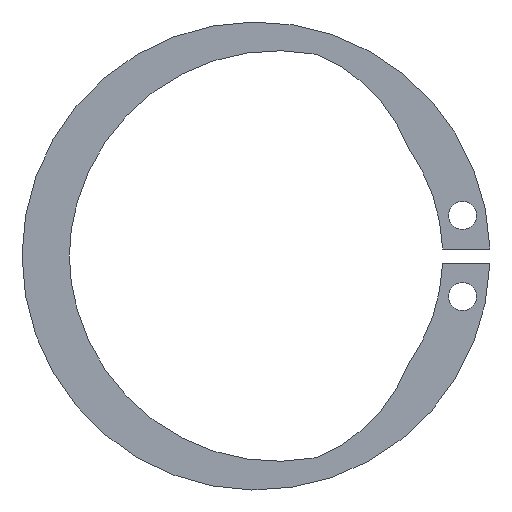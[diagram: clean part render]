
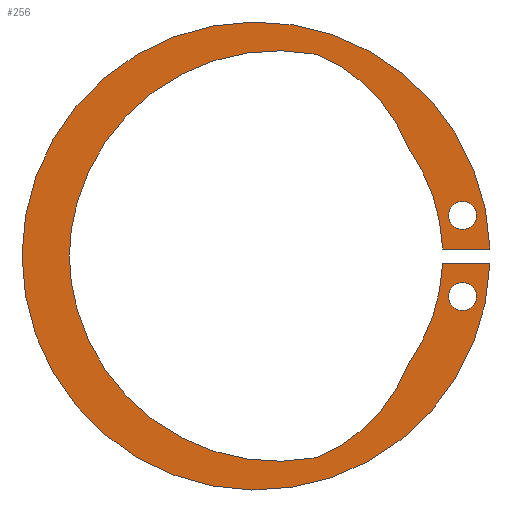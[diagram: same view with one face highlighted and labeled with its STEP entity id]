
A CAD part, front view. The second image highlights one B-rep face of the part: STEP entity #256.
In plain terms, the highlighted planar face has unit normal (0, -1, 0).
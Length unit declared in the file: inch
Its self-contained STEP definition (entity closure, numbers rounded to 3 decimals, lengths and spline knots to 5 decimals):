
#18=PLANE('',#310);
#21=LINE('',#417,#35);
#31=LINE('',#464,#45);
#35=VECTOR('',#335,0.3937);
#45=VECTOR('',#389,0.3937);
#51=FACE_BOUND('',#85,.T.);
#52=FACE_BOUND('',#86,.T.);
#66=FACE_OUTER_BOUND('',#84,.T.);
#84=EDGE_LOOP('',(#221,#222,#223,#224,#225,#226,#227,#228,#229,#230));
#85=EDGE_LOOP('',(#231));
#86=EDGE_LOOP('',(#232));
#88=CIRCLE('',#279,0.05);
#90=CIRCLE('',#282,0.05);
#91=CIRCLE('',#284,0.8355);
#93=CIRCLE('',#288,0.6665);
#95=CIRCLE('',#291,0.57967);
#97=CIRCLE('',#294,0.74404);
#99=CIRCLE('',#297,0.6665);
#101=CIRCLE('',#300,0.74404);
#103=CIRCLE('',#303,0.57967);
#105=CIRCLE('',#306,0.6665);
#108=VERTEX_POINT('',#399);
#110=VERTEX_POINT('',#404);
#111=VERTEX_POINT('',#407);
#112=VERTEX_POINT('',#408);
#115=VERTEX_POINT('',#416);
#117=VERTEX_POINT('',#422);
#119=VERTEX_POINT('',#428);
#121=VERTEX_POINT('',#434);
#123=VERTEX_POINT('',#440);
#125=VERTEX_POINT('',#446);
#127=VERTEX_POINT('',#452);
#129=VERTEX_POINT('',#458);
#132=EDGE_CURVE('',#108,#108,#88,.T.);
#134=EDGE_CURVE('',#110,#110,#90,.T.);
#135=EDGE_CURVE('',#111,#112,#91,.T.);
#139=EDGE_CURVE('',#115,#111,#21,.T.);
#142=EDGE_CURVE('',#117,#115,#93,.T.);
#145=EDGE_CURVE('',#119,#117,#95,.T.);
#148=EDGE_CURVE('',#121,#119,#97,.T.);
#151=EDGE_CURVE('',#123,#121,#99,.T.);
#154=EDGE_CURVE('',#125,#123,#101,.T.);
#157=EDGE_CURVE('',#127,#125,#103,.T.);
#160=EDGE_CURVE('',#129,#127,#105,.T.);
#163=EDGE_CURVE('',#112,#129,#31,.T.);
#221=ORIENTED_EDGE('',*,*,#163,.F.);
#222=ORIENTED_EDGE('',*,*,#135,.F.);
#223=ORIENTED_EDGE('',*,*,#139,.F.);
#224=ORIENTED_EDGE('',*,*,#142,.F.);
#225=ORIENTED_EDGE('',*,*,#145,.F.);
#226=ORIENTED_EDGE('',*,*,#148,.F.);
#227=ORIENTED_EDGE('',*,*,#151,.F.);
#228=ORIENTED_EDGE('',*,*,#154,.F.);
#229=ORIENTED_EDGE('',*,*,#157,.F.);
#230=ORIENTED_EDGE('',*,*,#160,.F.);
#231=ORIENTED_EDGE('',*,*,#132,.T.);
#232=ORIENTED_EDGE('',*,*,#134,.T.);
#256=ADVANCED_FACE('',(#66,#51,#52),#18,.F.);
#279=AXIS2_PLACEMENT_3D('',#400,#317,#318);
#282=AXIS2_PLACEMENT_3D('',#405,#323,#324);
#284=AXIS2_PLACEMENT_3D('',#409,#327,#328);
#288=AXIS2_PLACEMENT_3D('',#423,#340,#341);
#291=AXIS2_PLACEMENT_3D('',#429,#347,#348);
#294=AXIS2_PLACEMENT_3D('',#435,#354,#355);
#297=AXIS2_PLACEMENT_3D('',#441,#361,#362);
#300=AXIS2_PLACEMENT_3D('',#447,#368,#369);
#303=AXIS2_PLACEMENT_3D('',#453,#375,#376);
#306=AXIS2_PLACEMENT_3D('',#459,#382,#383);
#310=AXIS2_PLACEMENT_3D('',#467,#393,#394);
#317=DIRECTION('center_axis',(0.,1.,0.));
#318=DIRECTION('ref_axis',(1.,0.,0.));
#323=DIRECTION('center_axis',(0.,1.,0.));
#324=DIRECTION('ref_axis',(1.,0.,0.));
#327=DIRECTION('center_axis',(0.,1.,0.));
#328=DIRECTION('ref_axis',(0.999,0.,-0.033));
#335=DIRECTION('',(1.,0.,-0.017));
#340=DIRECTION('center_axis',(0.,-1.,0.));
#341=DIRECTION('ref_axis',(-0.999,0.,0.038));
#347=DIRECTION('center_axis',(0.,-1.,0.));
#348=DIRECTION('ref_axis',(-0.935,0.,0.354));
#354=DIRECTION('center_axis',(0.,-1.,0.));
#355=DIRECTION('ref_axis',(-0.184,0.,0.983));
#361=DIRECTION('center_axis',(0.,-1.,0.));
#362=DIRECTION('ref_axis',(0.96,0.,0.279));
#368=DIRECTION('center_axis',(0.,-1.,0.));
#369=DIRECTION('ref_axis',(1.,0.,-0.015));
#375=DIRECTION('center_axis',(0.,-1.,0.));
#376=DIRECTION('ref_axis',(-0.368,0.,-0.93));
#382=DIRECTION('center_axis',(0.,-1.,0.));
#383=DIRECTION('ref_axis',(-0.815,0.,-0.58));
#389=DIRECTION('',(-1.,0.,0.));
#393=DIRECTION('center_axis',(0.,1.,0.));
#394=DIRECTION('ref_axis',(0.,0.,1.));
#399=CARTESIAN_POINT('',(0.68741,0.,-0.14486));
#400=CARTESIAN_POINT('Origin',(0.73741,0.,-0.14486));
#404=CARTESIAN_POINT('',(0.68741,0.,0.14486));
#405=CARTESIAN_POINT('Origin',(0.73741,0.,0.14486));
#407=CARTESIAN_POINT('',(0.83504,0.,-0.02781));
#408=CARTESIAN_POINT('',(0.83513,0.,0.025));
#409=CARTESIAN_POINT('Origin',(0.,0.,0.));
#416=CARTESIAN_POINT('',(0.66603,0.,-0.025));
#417=CARTESIAN_POINT('',(0.66603,0.,-0.025));
#422=CARTESIAN_POINT('',(0.54302,0.,-0.38646));
#423=CARTESIAN_POINT('Origin',(0.,0.,0.));
#428=CARTESIAN_POINT('',(0.2141,0.,-0.72036));
#429=CARTESIAN_POINT('Origin',(0.00086,0.,-0.18134));
#434=CARTESIAN_POINT('',(-0.64002,0.,-0.18601));
#435=CARTESIAN_POINT('Origin',(0.07746,0.,0.01103));
#440=CARTESIAN_POINT('',(-0.64002,0.,0.18601));
#441=CARTESIAN_POINT('Origin',(0.,0.,0.));
#446=CARTESIAN_POINT('',(0.2141,0.,0.72036));
#447=CARTESIAN_POINT('Origin',(0.07746,0.,-0.01103));
#452=CARTESIAN_POINT('',(0.54302,0.,0.38646));
#453=CARTESIAN_POINT('Origin',(0.00086,0.,0.18134));
#458=CARTESIAN_POINT('',(0.66603,0.,0.025));
#459=CARTESIAN_POINT('Origin',(0.,0.,0.));
#464=CARTESIAN_POINT('',(0.83513,0.,0.025));
#467=CARTESIAN_POINT('Origin',(0.0293,0.,-0.00002));
